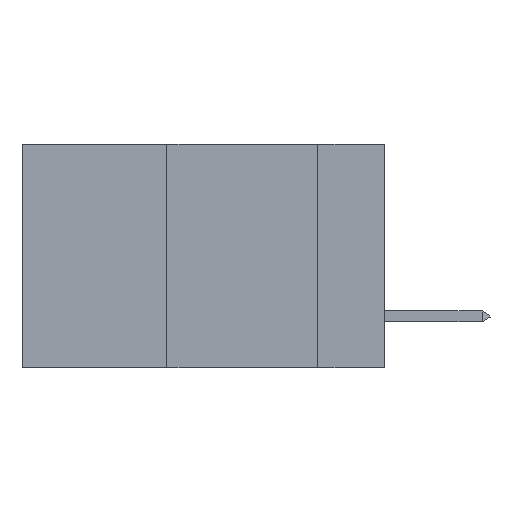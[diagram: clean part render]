
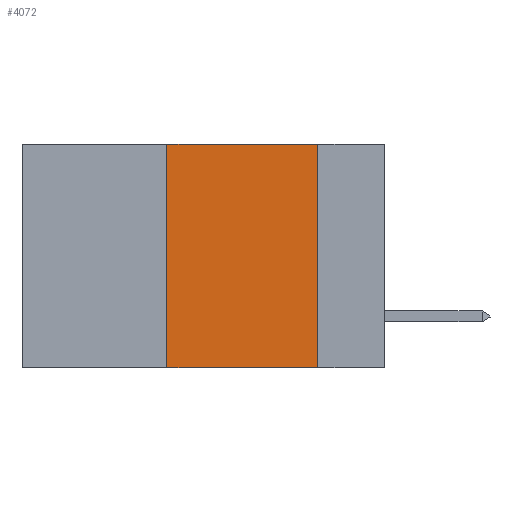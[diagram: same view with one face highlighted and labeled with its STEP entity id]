
A CAD part, left-side view. The second image highlights one B-rep face of the part: STEP entity #4072.
In plain terms, the highlighted planar face has unit normal (-1, 0, 0).
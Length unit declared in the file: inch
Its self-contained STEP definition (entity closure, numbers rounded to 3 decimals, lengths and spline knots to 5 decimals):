
#951 = VERTEX_POINT ( 'NONE', #2221 ) ;
#999 = CARTESIAN_POINT ( 'NONE',  ( 0., 0.11, 0. ) ) ;
#1533 = EDGE_CURVE ( 'NONE', #6655, #3035, #7773, .T. ) ;
#1570 = CARTESIAN_POINT ( 'NONE',  ( 0., 0.6, 0. ) ) ;
#2044 = ORIENTED_EDGE ( 'NONE', *, *, #9338, .F. ) ;
#2058 = CARTESIAN_POINT ( 'NONE',  ( 0., 0.36, 0. ) ) ;
#2128 = CARTESIAN_POINT ( 'NONE',  ( 0., 0.11, 0. ) ) ;
#2221 = CARTESIAN_POINT ( 'NONE',  ( 0., 0.36, -0.37 ) ) ;
#2318 = EDGE_LOOP ( 'NONE', ( #7560, #7681, #2044, #9920 ) ) ;
#2460 = DIRECTION ( 'NONE',  ( 0., 0., -1. ) ) ;
#2518 = DIRECTION ( 'NONE',  ( 0., 0., 1. ) ) ;
#3035 = VERTEX_POINT ( 'NONE', #999 ) ;
#3314 = VECTOR ( 'NONE', #3321, 39.37008 ) ;
#3321 = DIRECTION ( 'NONE',  ( 0., -1., 0. ) ) ;
#3440 = EDGE_CURVE ( 'NONE', #3035, #7393, #3646, .T. ) ;
#3624 = LINE ( 'NONE', #9666, #4973 ) ;
#3646 = LINE ( 'NONE', #2128, #5238 ) ;
#4037 = AXIS2_PLACEMENT_3D ( 'NONE', #7294, #6487, #2460 ) ;
#4072 = ADVANCED_FACE ( 'NONE', ( #7216 ), #8742, .F. ) ;
#4438 = CARTESIAN_POINT ( 'NONE',  ( 0., 0.6, -0.37 ) ) ;
#4973 = VECTOR ( 'NONE', #2518, 39.37008 ) ;
#5238 = VECTOR ( 'NONE', #6878, 39.37008 ) ;
#5877 = CARTESIAN_POINT ( 'NONE',  ( 0., 0.11, -0.37 ) ) ;
#6487 = DIRECTION ( 'NONE',  ( 1., 0., 0. ) ) ;
#6655 = VERTEX_POINT ( 'NONE', #2058 ) ;
#6878 = DIRECTION ( 'NONE',  ( 0., 0., -1. ) ) ;
#7089 = EDGE_CURVE ( 'NONE', #951, #7393, #8895, .T. ) ;
#7216 = FACE_OUTER_BOUND ( 'NONE', #2318, .T. ) ;
#7294 = CARTESIAN_POINT ( 'NONE',  ( 0., 0.6, 0. ) ) ;
#7393 = VERTEX_POINT ( 'NONE', #5877 ) ;
#7560 = ORIENTED_EDGE ( 'NONE', *, *, #3440, .F. ) ;
#7639 = DIRECTION ( 'NONE',  ( 0., -1., 0. ) ) ;
#7681 = ORIENTED_EDGE ( 'NONE', *, *, #1533, .F. ) ;
#7773 = LINE ( 'NONE', #1570, #3314 ) ;
#8742 = PLANE ( 'NONE',  #4037 ) ;
#8895 = LINE ( 'NONE', #4438, #9755 ) ;
#9338 = EDGE_CURVE ( 'NONE', #951, #6655, #3624, .T. ) ;
#9666 = CARTESIAN_POINT ( 'NONE',  ( 0., 0.36, 0. ) ) ;
#9755 = VECTOR ( 'NONE', #7639, 39.37008 ) ;
#9920 = ORIENTED_EDGE ( 'NONE', *, *, #7089, .T. ) ;
